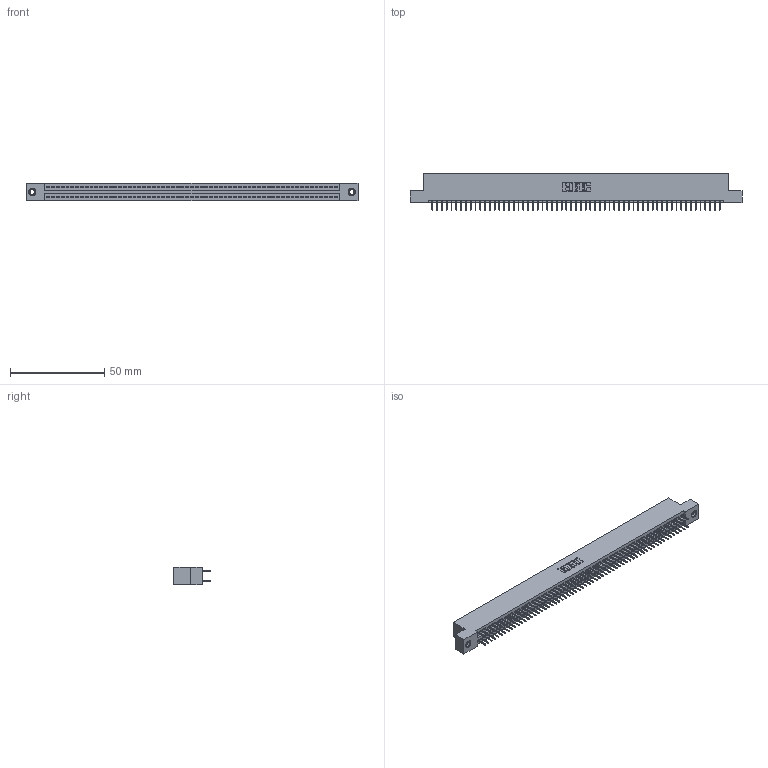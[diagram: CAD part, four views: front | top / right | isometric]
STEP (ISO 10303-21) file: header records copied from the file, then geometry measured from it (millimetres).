
FILE_DESCRIPTION (( 'STEP AP203' ), '1' );
FILE_NAME ('395-122-524-207.STEP', '2019-10-28T07:27:33', ( '' ), ( '' ), 'SwSTEP 2.0', 'SolidWorks 2016', '' );
FILE_SCHEMA (( 'CONFIG_CONTROL_DESIGN' ));
Length unit declared in the file: inch
Products named in the file (4): 345 Part_Flush Mounting Lugs - 0.156 Dia-TI; 345-292-001_345-293-124; 345-250-001_345-250-005-103; 395-122-524-207
Assembly tree (125 placements, depth 2):
  395-122-524-207
    345 Part_Flush Mounting Lugs - 0.156 Dia-TI
    345-292-001_345-293-124  x122
    345-250-001_345-250-005-103  x2
Bounding box: 176.15 x 19.35 x 9.4 mm (x, y, z)
Volume: 17089.5 mm3; surface area: 25169.7 mm2
Topology: 125 solids, 125 shells, 6774 faces, 19143 edges, 12266 vertices
Faces by surface type: plane 4870, cylinder 1888, cone 12, torus 4
Entity records: 46564 total; most frequent: CARTESIAN_POINT 7767, ORIENTED_EDGE 7694, DIRECTION 6853, EDGE_CURVE 3847, VECTOR 3455, LINE 3455, VERTEX_POINT 2556, AXIS2_PLACEMENT_3D 1699
